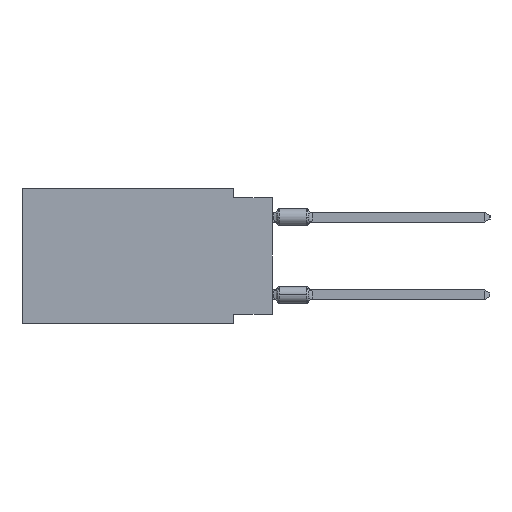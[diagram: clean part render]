
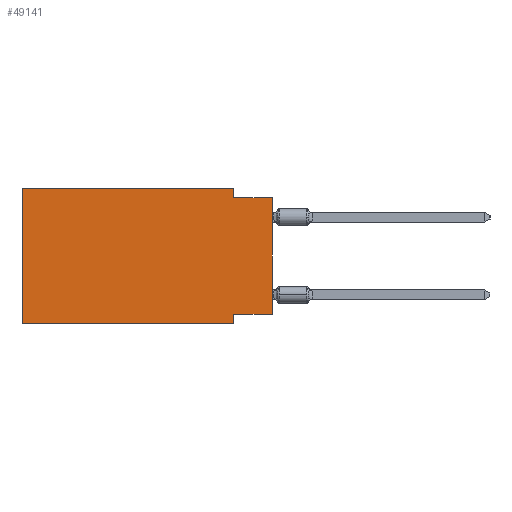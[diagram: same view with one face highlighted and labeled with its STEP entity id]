
A CAD part, left-side view. The second image highlights one B-rep face of the part: STEP entity #49141.
In plain terms, the highlighted planar face has unit normal (-1, 0, 0).
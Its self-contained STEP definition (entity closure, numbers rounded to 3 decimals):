
#1172 = DIRECTION ( 'NONE',  ( 1., 0., 0. ) ) ;
#1635 = EDGE_CURVE ( 'NONE', #11072, #44234, #45721, .T. ) ;
#2459 = CARTESIAN_POINT ( 'NONE',  ( 0., 2.54, -8.89 ) ) ;
#4771 = ORIENTED_EDGE ( 'NONE', *, *, #33523, .F. ) ;
#4774 = PLANE ( 'NONE',  #12601 ) ;
#5268 = EDGE_CURVE ( 'NONE', #46445, #19423, #43286, .T. ) ;
#5722 = EDGE_LOOP ( 'NONE', ( #48931, #38757, #53116, #31768, #4771, #20238, #31954, #26571 ) ) ;
#6253 = EDGE_CURVE ( 'NONE', #46445, #8787, #38208, .T. ) ;
#7022 = DIRECTION ( 'NONE',  ( 0., 0., 1. ) ) ;
#7554 = CARTESIAN_POINT ( 'NONE',  ( 0., 16.383, 0. ) ) ;
#8787 = VERTEX_POINT ( 'NONE', #39133 ) ;
#11072 = VERTEX_POINT ( 'NONE', #41967 ) ;
#12115 = VECTOR ( 'NONE', #22708, 1000. ) ;
#12311 = VECTOR ( 'NONE', #41219, 1000. ) ;
#12601 = AXIS2_PLACEMENT_3D ( 'NONE', #34690, #1172, #51258 ) ;
#13951 = DIRECTION ( 'NONE',  ( 0., 0., 1. ) ) ;
#15316 = CARTESIAN_POINT ( 'NONE',  ( 0., 16.383, 0. ) ) ;
#16400 = VERTEX_POINT ( 'NONE', #23909 ) ;
#16734 = CARTESIAN_POINT ( 'NONE',  ( 0., 2.54, -8.89 ) ) ;
#17265 = CARTESIAN_POINT ( 'NONE',  ( 0., 0., -0.635 ) ) ;
#18215 = EDGE_CURVE ( 'NONE', #16400, #19423, #27965, .T. ) ;
#19423 = VERTEX_POINT ( 'NONE', #17265 ) ;
#20238 = ORIENTED_EDGE ( 'NONE', *, *, #32916, .T. ) ;
#20563 = DIRECTION ( 'NONE',  ( 0., -1., 0. ) ) ;
#20613 = VECTOR ( 'NONE', #50717, 1000. ) ;
#21118 = VECTOR ( 'NONE', #13951, 1000. ) ;
#21171 = CARTESIAN_POINT ( 'NONE',  ( 0., 2.54, 0. ) ) ;
#21976 = LINE ( 'NONE', #21171, #20613 ) ;
#22292 = CARTESIAN_POINT ( 'NONE',  ( 0., 2.54, 0. ) ) ;
#22552 = VERTEX_POINT ( 'NONE', #16734 ) ;
#22708 = DIRECTION ( 'NONE',  ( 0., 0., -1. ) ) ;
#22726 = VECTOR ( 'NONE', #7022, 1000. ) ;
#23909 = CARTESIAN_POINT ( 'NONE',  ( 0., 2.54, -0.635 ) ) ;
#26571 = ORIENTED_EDGE ( 'NONE', *, *, #6253, .F. ) ;
#26699 = CARTESIAN_POINT ( 'NONE',  ( 0., 0., 0. ) ) ;
#27965 = LINE ( 'NONE', #31841, #12311 ) ;
#31366 = VECTOR ( 'NONE', #20563, 1000. ) ;
#31471 = LINE ( 'NONE', #52747, #35910 ) ;
#31768 = ORIENTED_EDGE ( 'NONE', *, *, #1635, .F. ) ;
#31841 = CARTESIAN_POINT ( 'NONE',  ( 0., 0., -0.635 ) ) ;
#31954 = ORIENTED_EDGE ( 'NONE', *, *, #46885, .F. ) ;
#32916 = EDGE_CURVE ( 'NONE', #36836, #22552, #31471, .T. ) ;
#33523 = EDGE_CURVE ( 'NONE', #36836, #11072, #41055, .T. ) ;
#33789 = DIRECTION ( 'NONE',  ( 0., 1., 0. ) ) ;
#34690 = CARTESIAN_POINT ( 'NONE',  ( 0., 16.383, 0. ) ) ;
#35910 = VECTOR ( 'NONE', #40048, 1000. ) ;
#36252 = LINE ( 'NONE', #2459, #12115 ) ;
#36836 = VERTEX_POINT ( 'NONE', #37377 ) ;
#37377 = CARTESIAN_POINT ( 'NONE',  ( 0., 16.383, -8.89 ) ) ;
#37721 = EDGE_CURVE ( 'NONE', #44234, #16400, #21976, .T. ) ;
#38208 = LINE ( 'NONE', #50618, #43238 ) ;
#38757 = ORIENTED_EDGE ( 'NONE', *, *, #18215, .F. ) ;
#39133 = CARTESIAN_POINT ( 'NONE',  ( 0., 2.54, -8.255 ) ) ;
#40048 = DIRECTION ( 'NONE',  ( 0., -1., 0. ) ) ;
#41055 = LINE ( 'NONE', #7554, #22726 ) ;
#41219 = DIRECTION ( 'NONE',  ( 0., -1., 0. ) ) ;
#41967 = CARTESIAN_POINT ( 'NONE',  ( 0., 16.383, 0. ) ) ;
#43238 = VECTOR ( 'NONE', #33789, 1000. ) ;
#43286 = LINE ( 'NONE', #26699, #21118 ) ;
#44234 = VERTEX_POINT ( 'NONE', #22292 ) ;
#45721 = LINE ( 'NONE', #15316, #31366 ) ;
#46445 = VERTEX_POINT ( 'NONE', #46549 ) ;
#46549 = CARTESIAN_POINT ( 'NONE',  ( 0., 0., -8.255 ) ) ;
#46885 = EDGE_CURVE ( 'NONE', #8787, #22552, #36252, .T. ) ;
#47382 = FACE_OUTER_BOUND ( 'NONE', #5722, .T. ) ;
#48931 = ORIENTED_EDGE ( 'NONE', *, *, #5268, .T. ) ;
#49141 = ADVANCED_FACE ( 'NONE', ( #47382 ), #4774, .F. ) ;
#50618 = CARTESIAN_POINT ( 'NONE',  ( 0., 0., -8.255 ) ) ;
#50717 = DIRECTION ( 'NONE',  ( 0., 0., -1. ) ) ;
#51258 = DIRECTION ( 'NONE',  ( 0., 0., -1. ) ) ;
#52747 = CARTESIAN_POINT ( 'NONE',  ( 0., 16.383, -8.89 ) ) ;
#53116 = ORIENTED_EDGE ( 'NONE', *, *, #37721, .F. ) ;
